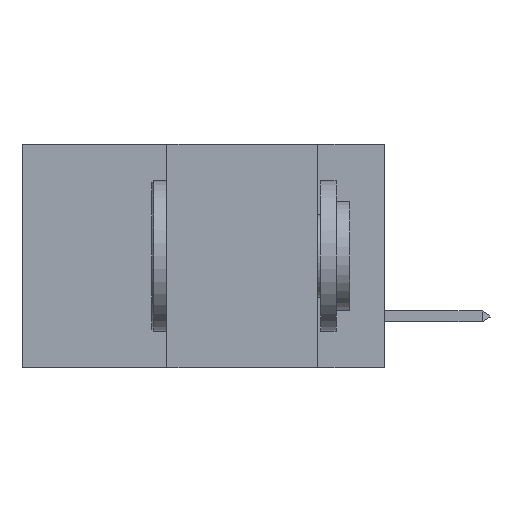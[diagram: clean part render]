
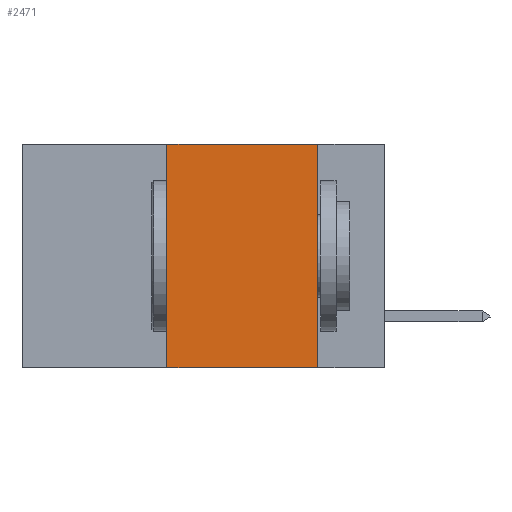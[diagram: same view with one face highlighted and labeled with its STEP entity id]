
A CAD part, left-side view. The second image highlights one B-rep face of the part: STEP entity #2471.
In plain terms, the highlighted planar face has unit normal (-1, 0, 0).
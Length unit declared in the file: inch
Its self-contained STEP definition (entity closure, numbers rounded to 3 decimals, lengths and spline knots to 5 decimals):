
#1491 = AXIS2_PLACEMENT_3D ( 'NONE', #17365, #4160, #8681 ) ;
#1808 = CARTESIAN_POINT ( 'NONE',  ( 0., 0.36, -0.37 ) ) ;
#2129 = LINE ( 'NONE', #17012, #3508 ) ;
#2188 = VERTEX_POINT ( 'NONE', #1808 ) ;
#2471 = ADVANCED_FACE ( 'NONE', ( #6426 ), #11583, .F. ) ;
#2542 = CARTESIAN_POINT ( 'NONE',  ( 0., 0.36, 0. ) ) ;
#2889 = CARTESIAN_POINT ( 'NONE',  ( 0., 0.36, 0. ) ) ;
#3006 = EDGE_CURVE ( 'NONE', #2188, #18381, #17569, .T. ) ;
#3187 = VECTOR ( 'NONE', #10257, 39.37008 ) ;
#3508 = VECTOR ( 'NONE', #18505, 39.37008 ) ;
#4160 = DIRECTION ( 'NONE',  ( 1., 0., 0. ) ) ;
#5495 = CARTESIAN_POINT ( 'NONE',  ( 0., 0.11, 0. ) ) ;
#5513 = LINE ( 'NONE', #14165, #13040 ) ;
#5585 = VECTOR ( 'NONE', #11867, 39.37008 ) ;
#6426 = FACE_OUTER_BOUND ( 'NONE', #8348, .T. ) ;
#8348 = EDGE_LOOP ( 'NONE', ( #11949, #15511, #9672, #17278 ) ) ;
#8681 = DIRECTION ( 'NONE',  ( 0., 0., -1. ) ) ;
#9672 = ORIENTED_EDGE ( 'NONE', *, *, #3006, .F. ) ;
#10176 = LINE ( 'NONE', #17493, #5585 ) ;
#10257 = DIRECTION ( 'NONE',  ( 0., 0., 1. ) ) ;
#11583 = PLANE ( 'NONE',  #1491 ) ;
#11867 = DIRECTION ( 'NONE',  ( 0., 0., -1. ) ) ;
#11949 = ORIENTED_EDGE ( 'NONE', *, *, #13923, .F. ) ;
#12196 = VERTEX_POINT ( 'NONE', #5495 ) ;
#13040 = VECTOR ( 'NONE', #18535, 39.37008 ) ;
#13248 = CARTESIAN_POINT ( 'NONE',  ( 0., 0.11, -0.37 ) ) ;
#13655 = EDGE_CURVE ( 'NONE', #18381, #12196, #2129, .T. ) ;
#13923 = EDGE_CURVE ( 'NONE', #12196, #17562, #10176, .T. ) ;
#14165 = CARTESIAN_POINT ( 'NONE',  ( 0., 0.6, -0.37 ) ) ;
#15511 = ORIENTED_EDGE ( 'NONE', *, *, #13655, .F. ) ;
#16029 = EDGE_CURVE ( 'NONE', #2188, #17562, #5513, .T. ) ;
#17012 = CARTESIAN_POINT ( 'NONE',  ( 0., 0.6, 0. ) ) ;
#17278 = ORIENTED_EDGE ( 'NONE', *, *, #16029, .T. ) ;
#17365 = CARTESIAN_POINT ( 'NONE',  ( 0., 0.6, 0. ) ) ;
#17493 = CARTESIAN_POINT ( 'NONE',  ( 0., 0.11, 0. ) ) ;
#17562 = VERTEX_POINT ( 'NONE', #13248 ) ;
#17569 = LINE ( 'NONE', #2889, #3187 ) ;
#18381 = VERTEX_POINT ( 'NONE', #2542 ) ;
#18505 = DIRECTION ( 'NONE',  ( 0., -1., 0. ) ) ;
#18535 = DIRECTION ( 'NONE',  ( 0., -1., 0. ) ) ;
